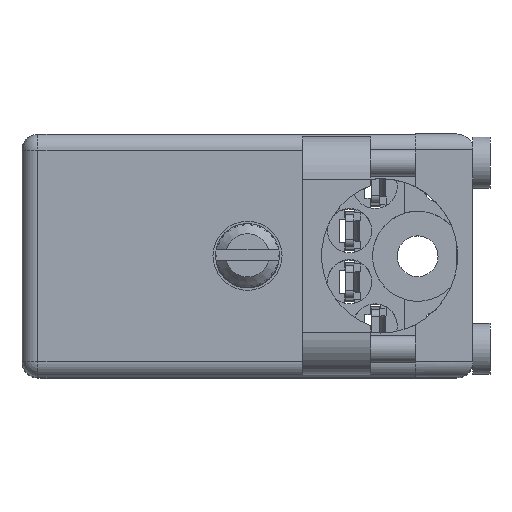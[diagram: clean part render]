
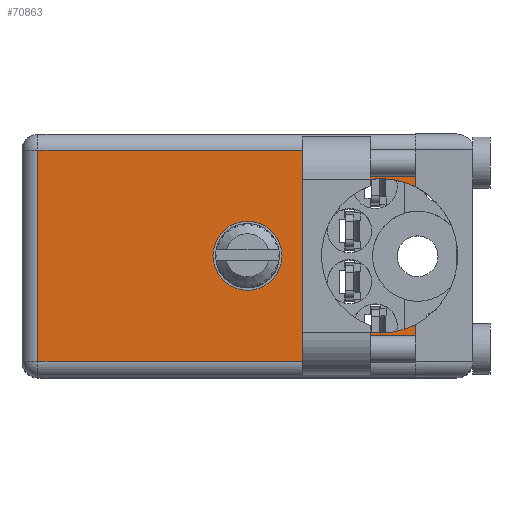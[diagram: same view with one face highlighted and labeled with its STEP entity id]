
A CAD part, top view. The second image highlights one B-rep face of the part: STEP entity #70863.
In plain terms, the highlighted face is planar.
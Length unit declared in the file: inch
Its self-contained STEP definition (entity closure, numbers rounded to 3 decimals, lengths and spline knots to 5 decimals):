
#872 = EDGE_LOOP ( 'NONE', ( #152954, #95407, #46634, #147454, #10137, #112673, #109776, #122784 ) ) ;
#4492 = AXIS2_PLACEMENT_3D ( 'NONE', #109927, #168602, #36988 ) ;
#8585 = CARTESIAN_POINT ( 'NONE',  ( 1.155, 0.906, -0.56029 ) ) ;
#9712 = CARTESIAN_POINT ( 'NONE',  ( 1.053, 0.906, -0.3575 ) ) ;
#10042 = DIRECTION ( 'NONE',  ( 1., 0., 0. ) ) ;
#10137 = ORIENTED_EDGE ( 'NONE', *, *, #183665, .F. ) ;
#10367 = CARTESIAN_POINT ( 'NONE',  ( 1.155, 0.906, 0. ) ) ;
#16399 = DIRECTION ( 'NONE',  ( 0., 1., 0. ) ) ;
#18998 = AXIS2_PLACEMENT_3D ( 'NONE', #120041, #16399, #130739 ) ;
#23180 = DIRECTION ( 'NONE',  ( 0., 1., 0. ) ) ;
#24126 = CARTESIAN_POINT ( 'NONE',  ( 1.053, 0.906, -0.1305 ) ) ;
#26405 = CARTESIAN_POINT ( 'NONE',  ( 0.047, 0.906, -0.668 ) ) ;
#27425 = ORIENTED_EDGE ( 'NONE', *, *, #42059, .F. ) ;
#29030 = AXIS2_PLACEMENT_3D ( 'NONE', #56237, #88769, #158039 ) ;
#29504 = CARTESIAN_POINT ( 'NONE',  ( 1.155, 0.906, -0.15471 ) ) ;
#36988 = DIRECTION ( 'NONE',  ( 0., 0., 1. ) ) ;
#37603 = VERTEX_POINT ( 'NONE', #24126 ) ;
#37628 = EDGE_CURVE ( 'NONE', #146167, #37603, #103337, .T. ) ;
#42059 = EDGE_CURVE ( 'NONE', #62396, #150977, #99467, .T. ) ;
#45139 = AXIS2_PLACEMENT_3D ( 'NONE', #9712, #23180, #152896 ) ;
#45780 = EDGE_CURVE ( 'NONE', #37603, #101236, #53593, .T. ) ;
#45914 = ORIENTED_EDGE ( 'NONE', *, *, #131076, .F. ) ;
#46634 = ORIENTED_EDGE ( 'NONE', *, *, #111036, .T. ) ;
#50550 = CARTESIAN_POINT ( 'NONE',  ( 1.053, 0.906, -0.5845 ) ) ;
#51239 = DIRECTION ( 'NONE',  ( 0., 0., 1. ) ) ;
#53125 = DIRECTION ( 'NONE',  ( 0., 1., 0. ) ) ;
#53153 = FACE_BOUND ( 'NONE', #176553, .T. ) ;
#53593 = CIRCLE ( 'NONE', #29030, 0.227 ) ;
#55007 = CARTESIAN_POINT ( 'NONE',  ( 1.053, 0.906, -0.3575 ) ) ;
#55192 = CARTESIAN_POINT ( 'NONE',  ( 0.6625, 0.906, -0.459 ) ) ;
#56237 = CARTESIAN_POINT ( 'NONE',  ( 1.053, 0.906, -0.3575 ) ) ;
#62396 = VERTEX_POINT ( 'NONE', #55192 ) ;
#67511 = DIRECTION ( 'NONE',  ( 0., 0., 1. ) ) ;
#69163 = EDGE_CURVE ( 'NONE', #109116, #78584, #138809, .T. ) ;
#70863 = ADVANCED_FACE ( 'NONE', ( #96320, #53153 ), #169386, .T. ) ;
#72021 = DIRECTION ( 'NONE',  ( 0., 1., 0. ) ) ;
#72668 = DIRECTION ( 'NONE',  ( 0., 0., 1. ) ) ;
#73928 = CARTESIAN_POINT ( 'NONE',  ( 1.155, 0.906, -0.047 ) ) ;
#78584 = VERTEX_POINT ( 'NONE', #73928 ) ;
#81294 = VERTEX_POINT ( 'NONE', #8585 ) ;
#81537 = AXIS2_PLACEMENT_3D ( 'NONE', #140524, #72021, #67511 ) ;
#83810 = CIRCLE ( 'NONE', #18998, 0.1015 ) ;
#86098 = CARTESIAN_POINT ( 'NONE',  ( 1.155, 0.906, 0. ) ) ;
#88769 = DIRECTION ( 'NONE',  ( 0., 1., 0. ) ) ;
#91362 = DIRECTION ( 'NONE',  ( -1., 0., 0. ) ) ;
#95407 = ORIENTED_EDGE ( 'NONE', *, *, #110718, .T. ) ;
#96320 = FACE_OUTER_BOUND ( 'NONE', #872, .T. ) ;
#97219 = CARTESIAN_POINT ( 'NONE',  ( 1.155, 0.906, -0.668 ) ) ;
#99467 = CIRCLE ( 'NONE', #4492, 0.1015 ) ;
#101236 = VERTEX_POINT ( 'NONE', #29504 ) ;
#102164 = VECTOR ( 'NONE', #72668, 39.37008 ) ;
#103337 = CIRCLE ( 'NONE', #45139, 0.227 ) ;
#109112 = AXIS2_PLACEMENT_3D ( 'NONE', #55007, #53125, #51239 ) ;
#109116 = VERTEX_POINT ( 'NONE', #116530 ) ;
#109318 = DIRECTION ( 'NONE',  ( 0., 0., 1. ) ) ;
#109358 = VERTEX_POINT ( 'NONE', #97219 ) ;
#109776 = ORIENTED_EDGE ( 'NONE', *, *, #37628, .F. ) ;
#109927 = CARTESIAN_POINT ( 'NONE',  ( 0.6625, 0.906, -0.3575 ) ) ;
#109933 = CARTESIAN_POINT ( 'NONE',  ( 1.155, 0.906, -0.047 ) ) ;
#110718 = EDGE_CURVE ( 'NONE', #109358, #132343, #134614, .T. ) ;
#111036 = EDGE_CURVE ( 'NONE', #132343, #109116, #143841, .T. ) ;
#112163 = CARTESIAN_POINT ( 'NONE',  ( 0.047, 0.906, -0.715 ) ) ;
#112673 = ORIENTED_EDGE ( 'NONE', *, *, #45780, .F. ) ;
#113326 = VECTOR ( 'NONE', #109318, 39.37008 ) ;
#114026 = DIRECTION ( 'NONE',  ( 0., 0., 1. ) ) ;
#116530 = CARTESIAN_POINT ( 'NONE',  ( 0.047, 0.906, -0.047 ) ) ;
#116787 = LINE ( 'NONE', #86098, #102164 ) ;
#120041 = CARTESIAN_POINT ( 'NONE',  ( 0.6625, 0.906, -0.3575 ) ) ;
#122420 = CARTESIAN_POINT ( 'NONE',  ( 0.6625, 0.906, -0.256 ) ) ;
#122784 = ORIENTED_EDGE ( 'NONE', *, *, #156593, .F. ) ;
#126571 = LINE ( 'NONE', #10367, #113326 ) ;
#130739 = DIRECTION ( 'NONE',  ( 0., 0., 1. ) ) ;
#130807 = EDGE_CURVE ( 'NONE', #109358, #81294, #116787, .T. ) ;
#131076 = EDGE_CURVE ( 'NONE', #150977, #62396, #83810, .T. ) ;
#132343 = VERTEX_POINT ( 'NONE', #26405 ) ;
#132516 = VECTOR ( 'NONE', #114026, 39.37008 ) ;
#134614 = LINE ( 'NONE', #162511, #175626 ) ;
#138809 = LINE ( 'NONE', #109933, #148890 ) ;
#140524 = CARTESIAN_POINT ( 'NONE',  ( 0., 0.906, -0.715 ) ) ;
#143841 = LINE ( 'NONE', #112163, #132516 ) ;
#146167 = VERTEX_POINT ( 'NONE', #50550 ) ;
#147454 = ORIENTED_EDGE ( 'NONE', *, *, #69163, .T. ) ;
#148890 = VECTOR ( 'NONE', #10042, 39.37008 ) ;
#149056 = CIRCLE ( 'NONE', #109112, 0.227 ) ;
#150977 = VERTEX_POINT ( 'NONE', #122420 ) ;
#152896 = DIRECTION ( 'NONE',  ( 0., 0., 1. ) ) ;
#152954 = ORIENTED_EDGE ( 'NONE', *, *, #130807, .F. ) ;
#156593 = EDGE_CURVE ( 'NONE', #81294, #146167, #149056, .T. ) ;
#158039 = DIRECTION ( 'NONE',  ( 0., 0., 1. ) ) ;
#162511 = CARTESIAN_POINT ( 'NONE',  ( 0., 0.906, -0.668 ) ) ;
#168602 = DIRECTION ( 'NONE',  ( 0., 1., 0. ) ) ;
#169386 = PLANE ( 'NONE',  #81537 ) ;
#175626 = VECTOR ( 'NONE', #91362, 39.37008 ) ;
#176553 = EDGE_LOOP ( 'NONE', ( #45914, #27425 ) ) ;
#183665 = EDGE_CURVE ( 'NONE', #101236, #78584, #126571, .T. ) ;
